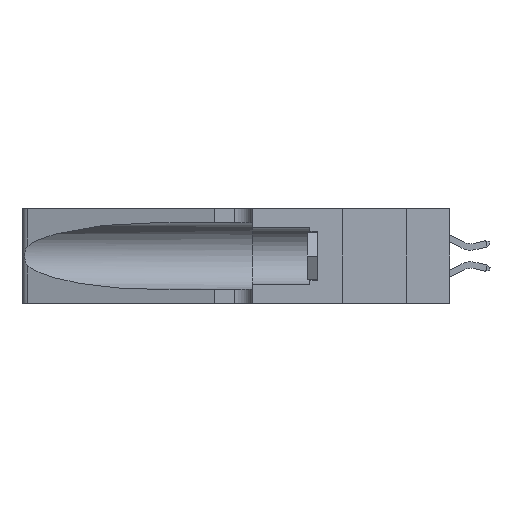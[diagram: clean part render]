
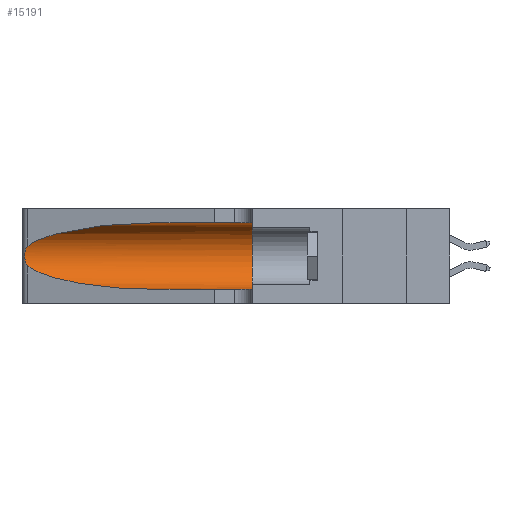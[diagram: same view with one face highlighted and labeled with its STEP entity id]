
A CAD part, left-side view. The second image highlights one B-rep face of the part: STEP entity #15191.
In plain terms, the highlighted cylindrical face has radius 3.308 mm (diameter 6.617 mm), a partial arc.
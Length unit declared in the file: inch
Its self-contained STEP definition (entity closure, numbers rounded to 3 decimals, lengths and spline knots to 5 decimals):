
#786 = CARTESIAN_POINT ( 'NONE',  ( 0.1305, 1.61858, 0.31525 ) ) ;
#1387 = CARTESIAN_POINT ( 'NONE',  ( 0.25487, 1.22718, 0.14631 ) ) ;
#1634 = CARTESIAN_POINT ( 'NONE',  ( 0.25639, 1.23184, 0.21858 ) ) ;
#2402 = AXIS2_PLACEMENT_3D ( 'NONE', #18499, #8776, #20152 ) ;
#2621 = B_SPLINE_CURVE_WITH_KNOTS ( 'NONE', 3,
 ( #3218, #12993, #1634, #13071, #3285, #14726, #4953, #16341, #6605, #17957, #8229, #19590, #9848, #8447 ),
 .UNSPECIFIED., .F., .F.,
 ( 4, 2, 2, 2, 2, 2, 4 ),
 ( 0., 0.00027, 0.00053, 0.00107, 0.0016, 0.00187, 0.00214 ),
 .UNSPECIFIED. ) ;
#3026 = ORIENTED_EDGE ( 'NONE', *, *, #13940, .T. ) ;
#3035 = ORIENTED_EDGE ( 'NONE', *, *, #17536, .T. ) ;
#3218 = CARTESIAN_POINT ( 'NONE',  ( 0.25487, 1.22718, 0.22369 ) ) ;
#3285 = CARTESIAN_POINT ( 'NONE',  ( 0.25854, 1.2359, 0.20912 ) ) ;
#3744 = FACE_OUTER_BOUND ( 'NONE', #4690, .T. ) ;
#4206 =( BOUNDED_CURVE ( )  B_SPLINE_CURVE ( 3, ( #1387, #11162, #9533, #12825 ),
 .UNSPECIFIED., .F., .F. ) 
 B_SPLINE_CURVE_WITH_KNOTS ( ( 4, 4 ),
 ( 3.44316, 4.71239 ),
 .UNSPECIFIED. ) 
 CURVE ( )  GEOMETRIC_REPRESENTATION_ITEM ( )  RATIONAL_B_SPLINE_CURVE ( ( 1., 0.87, 0.87, 1. ) ) 
 REPRESENTATION_ITEM ( '' )  );
#4408 = ORIENTED_EDGE ( 'NONE', *, *, #7665, .F. ) ;
#4690 = EDGE_LOOP ( 'NONE', ( #3026, #3035, #6024, #8679, #4408, #5397 ) ) ;
#4953 = CARTESIAN_POINT ( 'NONE',  ( 0.26075, 1.23896, 0.19203 ) ) ;
#5090 = CARTESIAN_POINT ( 'NONE',  ( 0.1305, 0.72297, 0.31525 ) ) ;
#5392 = DIRECTION ( 'NONE',  ( 0., -1., 0. ) ) ;
#5397 = ORIENTED_EDGE ( 'NONE', *, *, #12816, .F. ) ;
#6024 = ORIENTED_EDGE ( 'NONE', *, *, #9842, .T. ) ;
#6605 = CARTESIAN_POINT ( 'NONE',  ( 0.26017, 1.23833, 0.17102 ) ) ;
#6764 = VECTOR ( 'NONE', #11054, 39.37008 ) ;
#7041 = DIRECTION ( 'NONE',  ( 0., 0., -1. ) ) ;
#7277 = LINE ( 'NONE', #9416, #6764 ) ;
#7665 = EDGE_CURVE ( 'NONE', #18756, #19075, #14918, .T. ) ;
#8229 = CARTESIAN_POINT ( 'NONE',  ( 0.25789, 1.23486, 0.15765 ) ) ;
#8373 = CARTESIAN_POINT ( 'NONE',  ( 0.25487, 1.22718, 0.22369 ) ) ;
#8447 = CARTESIAN_POINT ( 'NONE',  ( 0.25487, 1.22718, 0.14631 ) ) ;
#8501 = VERTEX_POINT ( 'NONE', #12608 ) ;
#8679 = ORIENTED_EDGE ( 'NONE', *, *, #11143, .T. ) ;
#8776 = DIRECTION ( 'NONE',  ( 0., 1., 0. ) ) ;
#8975 = DIRECTION ( 'NONE',  ( 0., -1., 0. ) ) ;
#9209 = CARTESIAN_POINT ( 'NONE',  ( 0.1305, 0.72297, 0.05475 ) ) ;
#9416 = CARTESIAN_POINT ( 'NONE',  ( 0.1305, 1.61858, 0.05475 ) ) ;
#9533 = CARTESIAN_POINT ( 'NONE',  ( 0.18966, 0.96281, 0.05475 ) ) ;
#9842 = EDGE_CURVE ( 'NONE', #16285, #14319, #4206, .T. ) ;
#9848 = CARTESIAN_POINT ( 'NONE',  ( 0.25555, 1.22993, 0.14849 ) ) ;
#10037 = CARTESIAN_POINT ( 'NONE',  ( 0.25487, 1.22718, 0.14631 ) ) ;
#11054 = DIRECTION ( 'NONE',  ( 0., -1., 0. ) ) ;
#11143 = EDGE_CURVE ( 'NONE', #14319, #19075, #7277, .T. ) ;
#11162 = CARTESIAN_POINT ( 'NONE',  ( 0.2373, 1.15595, 0.08982 ) ) ;
#11386 = CYLINDRICAL_SURFACE ( 'NONE', #17112, 0.13025 ) ;
#11557 = CARTESIAN_POINT ( 'NONE',  ( 0.18966, 0.96281, 0.31525 ) ) ;
#11861 = CARTESIAN_POINT ( 'NONE',  ( 0.1305, 1.61858, 0.185 ) ) ;
#12608 = CARTESIAN_POINT ( 'NONE',  ( 0.1305, 0.72297, 0.31525 ) ) ;
#12816 = EDGE_CURVE ( 'NONE', #8501, #18756, #18879, .T. ) ;
#12825 = CARTESIAN_POINT ( 'NONE',  ( 0.1305, 0.72297, 0.05475 ) ) ;
#12993 = CARTESIAN_POINT ( 'NONE',  ( 0.25555, 1.22994, 0.2215 ) ) ;
#13071 = CARTESIAN_POINT ( 'NONE',  ( 0.25787, 1.23484, 0.2124 ) ) ;
#13559 = VECTOR ( 'NONE', #8975, 39.37008 ) ;
#13940 = EDGE_CURVE ( 'NONE', #8501, #16105, #17758, .T. ) ;
#14319 = VERTEX_POINT ( 'NONE', #9209 ) ;
#14726 = CARTESIAN_POINT ( 'NONE',  ( 0.26018, 1.23835, 0.19895 ) ) ;
#14918 = CIRCLE ( 'NONE', #2402, 0.13025 ) ;
#15191 = ADVANCED_FACE ( 'NONE', ( #3744 ), #11386, .F. ) ;
#16105 = VERTEX_POINT ( 'NONE', #16118 ) ;
#16118 = CARTESIAN_POINT ( 'NONE',  ( 0.25487, 1.22718, 0.22369 ) ) ;
#16184 = CARTESIAN_POINT ( 'NONE',  ( 0.1305, 0.35, 0.05475 ) ) ;
#16285 = VERTEX_POINT ( 'NONE', #10037 ) ;
#16341 = CARTESIAN_POINT ( 'NONE',  ( 0.26075, 1.23896, 0.178 ) ) ;
#17112 = AXIS2_PLACEMENT_3D ( 'NONE', #11861, #5392, #7041 ) ;
#17536 = EDGE_CURVE ( 'NONE', #16105, #16285, #2621, .T. ) ;
#17758 =( BOUNDED_CURVE ( )  B_SPLINE_CURVE ( 3, ( #5090, #11557, #18097, #8373 ),
 .UNSPECIFIED., .F., .F. ) 
 B_SPLINE_CURVE_WITH_KNOTS ( ( 4, 4 ),
 ( 1.5708, 2.84003 ),
 .UNSPECIFIED. ) 
 CURVE ( )  GEOMETRIC_REPRESENTATION_ITEM ( )  RATIONAL_B_SPLINE_CURVE ( ( 1., 0.87, 0.87, 1. ) ) 
 REPRESENTATION_ITEM ( '' )  );
#17957 = CARTESIAN_POINT ( 'NONE',  ( 0.25856, 1.23593, 0.16098 ) ) ;
#18097 = CARTESIAN_POINT ( 'NONE',  ( 0.2373, 1.15595, 0.28018 ) ) ;
#18499 = CARTESIAN_POINT ( 'NONE',  ( 0.1305, 0.35, 0.185 ) ) ;
#18756 = VERTEX_POINT ( 'NONE', #20311 ) ;
#18879 = LINE ( 'NONE', #786, #13559 ) ;
#19075 = VERTEX_POINT ( 'NONE', #16184 ) ;
#19590 = CARTESIAN_POINT ( 'NONE',  ( 0.25639, 1.23186, 0.15144 ) ) ;
#20152 = DIRECTION ( 'NONE',  ( 0., 0., 1. ) ) ;
#20311 = CARTESIAN_POINT ( 'NONE',  ( 0.1305, 0.35, 0.31525 ) ) ;
